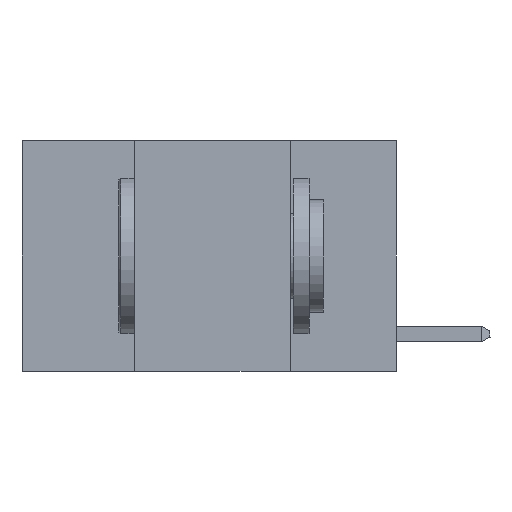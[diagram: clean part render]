
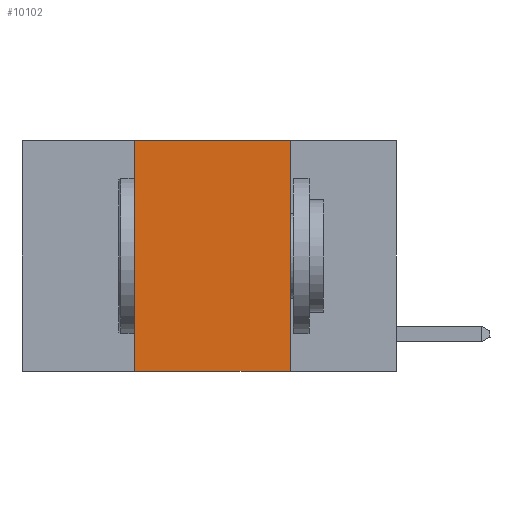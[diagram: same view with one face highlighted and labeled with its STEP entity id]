
A CAD part, left-side view. The second image highlights one B-rep face of the part: STEP entity #10102.
In plain terms, the highlighted planar face has unit normal (-1, 0, 0).
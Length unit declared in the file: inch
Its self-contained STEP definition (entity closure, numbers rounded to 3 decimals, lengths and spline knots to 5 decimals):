
#617 = CARTESIAN_POINT ( 'NONE',  ( 0., 0.6, -0.37 ) ) ;
#888 = LINE ( 'NONE', #2332, #3349 ) ;
#1094 = CARTESIAN_POINT ( 'NONE',  ( 0., 0.17, 0. ) ) ;
#1433 = ORIENTED_EDGE ( 'NONE', *, *, #5178, .F. ) ;
#1521 = VECTOR ( 'NONE', #10290, 39.37008 ) ;
#1622 = CARTESIAN_POINT ( 'NONE',  ( 0., 0.17, 0. ) ) ;
#1680 = EDGE_CURVE ( 'NONE', #2162, #1998, #888, .T. ) ;
#1953 = LINE ( 'NONE', #617, #1521 ) ;
#1998 = VERTEX_POINT ( 'NONE', #12285 ) ;
#2162 = VERTEX_POINT ( 'NONE', #4753 ) ;
#2332 = CARTESIAN_POINT ( 'NONE',  ( 0., 0.42, 0. ) ) ;
#3349 = VECTOR ( 'NONE', #17435, 39.37008 ) ;
#3532 = DIRECTION ( 'NONE',  ( 1., 0., 0. ) ) ;
#4753 = CARTESIAN_POINT ( 'NONE',  ( 0., 0.42, -0.37 ) ) ;
#5158 = AXIS2_PLACEMENT_3D ( 'NONE', #21870, #3532, #16764 ) ;
#5178 = EDGE_CURVE ( 'NONE', #1998, #21322, #20851, .T. ) ;
#7126 = ORIENTED_EDGE ( 'NONE', *, *, #1680, .F. ) ;
#7874 = DIRECTION ( 'NONE',  ( 0., 0., -1. ) ) ;
#8121 = VERTEX_POINT ( 'NONE', #17362 ) ;
#8220 = VECTOR ( 'NONE', #9205, 39.37008 ) ;
#9205 = DIRECTION ( 'NONE',  ( 0., -1., 0. ) ) ;
#10102 = ADVANCED_FACE ( 'NONE', ( #13552 ), #20300, .F. ) ;
#10290 = DIRECTION ( 'NONE',  ( 0., -1., 0. ) ) ;
#12285 = CARTESIAN_POINT ( 'NONE',  ( 0., 0.42, 0. ) ) ;
#13552 = FACE_OUTER_BOUND ( 'NONE', #15483, .T. ) ;
#14194 = ORIENTED_EDGE ( 'NONE', *, *, #15430, .T. ) ;
#15430 = EDGE_CURVE ( 'NONE', #2162, #8121, #1953, .T. ) ;
#15483 = EDGE_LOOP ( 'NONE', ( #18054, #1433, #7126, #14194 ) ) ;
#16764 = DIRECTION ( 'NONE',  ( 0., 0., -1. ) ) ;
#17362 = CARTESIAN_POINT ( 'NONE',  ( 0., 0.17, -0.37 ) ) ;
#17435 = DIRECTION ( 'NONE',  ( 0., 0., 1. ) ) ;
#17894 = VECTOR ( 'NONE', #7874, 39.37008 ) ;
#18054 = ORIENTED_EDGE ( 'NONE', *, *, #18417, .F. ) ;
#18417 = EDGE_CURVE ( 'NONE', #21322, #8121, #20075, .T. ) ;
#20075 = LINE ( 'NONE', #1094, #17894 ) ;
#20300 = PLANE ( 'NONE',  #5158 ) ;
#20851 = LINE ( 'NONE', #21078, #8220 ) ;
#21078 = CARTESIAN_POINT ( 'NONE',  ( 0., 0.6, 0. ) ) ;
#21322 = VERTEX_POINT ( 'NONE', #1622 ) ;
#21870 = CARTESIAN_POINT ( 'NONE',  ( 0., 0.6, 0. ) ) ;
